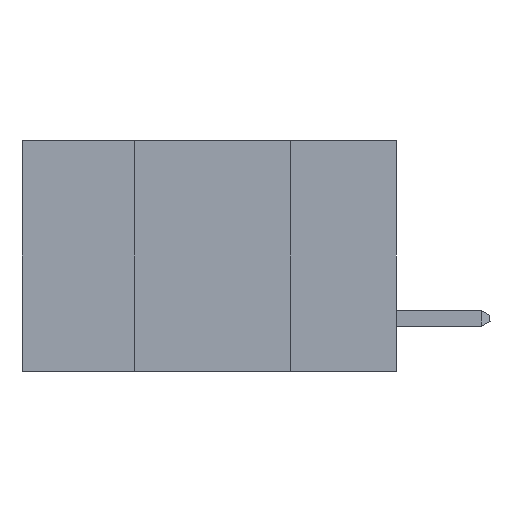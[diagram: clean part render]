
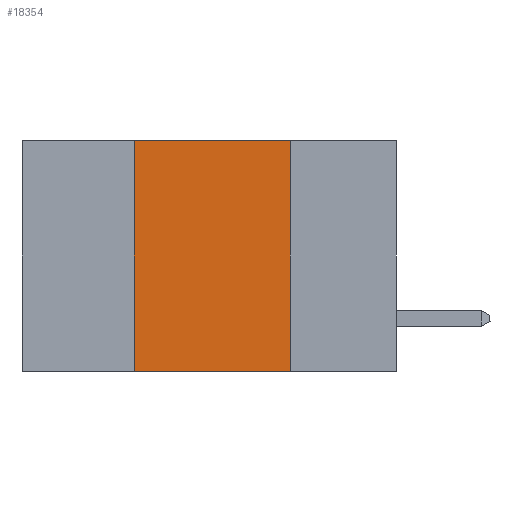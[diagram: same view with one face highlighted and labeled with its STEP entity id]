
A CAD part, left-side view. The second image highlights one B-rep face of the part: STEP entity #18354.
In plain terms, the highlighted planar face has unit normal (-1, 0, 0).
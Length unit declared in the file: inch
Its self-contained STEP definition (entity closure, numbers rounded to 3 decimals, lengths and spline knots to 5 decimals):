
#133 = ORIENTED_EDGE ( 'NONE', *, *, #5036, .F. ) ;
#1006 = DIRECTION ( 'NONE',  ( 0., 0., -1. ) ) ;
#2243 = ORIENTED_EDGE ( 'NONE', *, *, #9217, .T. ) ;
#4284 = DIRECTION ( 'NONE',  ( 0., -1., 0. ) ) ;
#4610 = ORIENTED_EDGE ( 'NONE', *, *, #5432, .F. ) ;
#5002 = CARTESIAN_POINT ( 'NONE',  ( 0., 0.42, 0. ) ) ;
#5036 = EDGE_CURVE ( 'NONE', #7950, #17270, #5988, .T. ) ;
#5192 = PLANE ( 'NONE',  #11980 ) ;
#5432 = EDGE_CURVE ( 'NONE', #17270, #7444, #6198, .T. ) ;
#5917 = DIRECTION ( 'NONE',  ( 0., -1., 0. ) ) ;
#5988 = LINE ( 'NONE', #10520, #9420 ) ;
#6050 = VECTOR ( 'NONE', #4284, 39.37008 ) ;
#6198 = LINE ( 'NONE', #16003, #17888 ) ;
#6923 = CARTESIAN_POINT ( 'NONE',  ( 0., 0.42, -0.37 ) ) ;
#7237 = CARTESIAN_POINT ( 'NONE',  ( 0., 0.17, 0. ) ) ;
#7444 = VERTEX_POINT ( 'NONE', #7237 ) ;
#7903 = EDGE_CURVE ( 'NONE', #7444, #17388, #9572, .T. ) ;
#7950 = VERTEX_POINT ( 'NONE', #6923 ) ;
#9217 = EDGE_CURVE ( 'NONE', #7950, #17388, #14508, .T. ) ;
#9420 = VECTOR ( 'NONE', #13682, 39.37008 ) ;
#9572 = LINE ( 'NONE', #11557, #14606 ) ;
#9906 = CARTESIAN_POINT ( 'NONE',  ( 0., 0.17, -0.37 ) ) ;
#10520 = CARTESIAN_POINT ( 'NONE',  ( 0., 0.42, 0. ) ) ;
#11557 = CARTESIAN_POINT ( 'NONE',  ( 0., 0.17, 0. ) ) ;
#11980 = AXIS2_PLACEMENT_3D ( 'NONE', #15433, #16908, #1006 ) ;
#13682 = DIRECTION ( 'NONE',  ( 0., 0., 1. ) ) ;
#14508 = LINE ( 'NONE', #17500, #6050 ) ;
#14606 = VECTOR ( 'NONE', #17360, 39.37008 ) ;
#15416 = FACE_OUTER_BOUND ( 'NONE', #17219, .T. ) ;
#15433 = CARTESIAN_POINT ( 'NONE',  ( 0., 0.6, 0. ) ) ;
#15697 = ORIENTED_EDGE ( 'NONE', *, *, #7903, .F. ) ;
#16003 = CARTESIAN_POINT ( 'NONE',  ( 0., 0.6, 0. ) ) ;
#16908 = DIRECTION ( 'NONE',  ( 1., 0., 0. ) ) ;
#17219 = EDGE_LOOP ( 'NONE', ( #15697, #4610, #133, #2243 ) ) ;
#17270 = VERTEX_POINT ( 'NONE', #5002 ) ;
#17360 = DIRECTION ( 'NONE',  ( 0., 0., -1. ) ) ;
#17388 = VERTEX_POINT ( 'NONE', #9906 ) ;
#17500 = CARTESIAN_POINT ( 'NONE',  ( 0., 0.6, -0.37 ) ) ;
#17888 = VECTOR ( 'NONE', #5917, 39.37008 ) ;
#18354 = ADVANCED_FACE ( 'NONE', ( #15416 ), #5192, .F. ) ;
